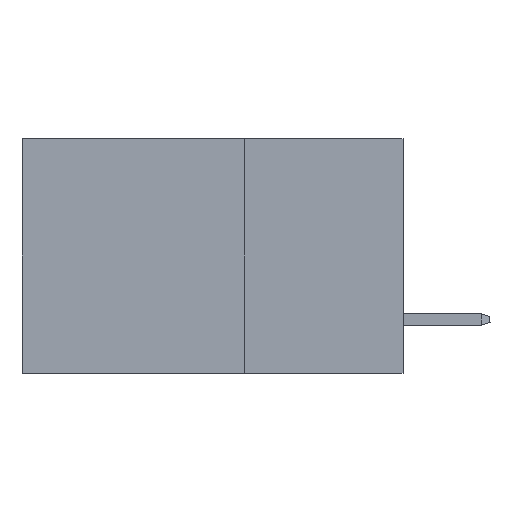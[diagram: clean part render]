
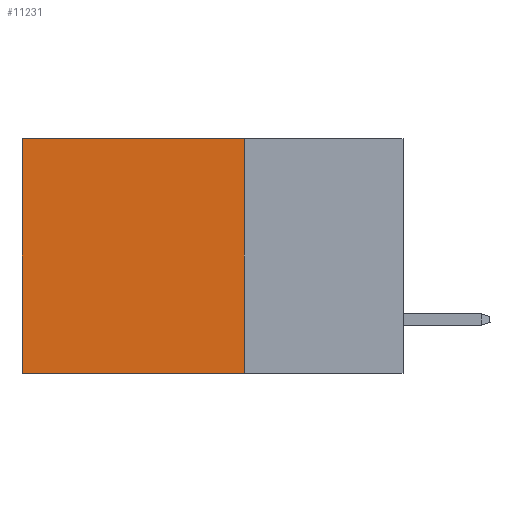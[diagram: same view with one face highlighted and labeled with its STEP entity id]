
A CAD part, left-side view. The second image highlights one B-rep face of the part: STEP entity #11231.
In plain terms, the highlighted planar face has unit normal (-1, 0, 0).
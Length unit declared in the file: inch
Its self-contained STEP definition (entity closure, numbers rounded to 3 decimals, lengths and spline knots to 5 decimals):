
#786 = DIRECTION ( 'NONE',  ( 0., 1., 0. ) ) ;
#881 = CARTESIAN_POINT ( 'NONE',  ( 0.2875, 0.25, 0. ) ) ;
#2865 = ORIENTED_EDGE ( 'NONE', *, *, #5326, .T. ) ;
#2967 = CARTESIAN_POINT ( 'NONE',  ( 0.2875, 0.25, 0. ) ) ;
#3061 = DIRECTION ( 'NONE',  ( 0., 0., -1. ) ) ;
#3342 = EDGE_CURVE ( 'NONE', #11267, #6676, #10036, .T. ) ;
#4133 = EDGE_CURVE ( 'NONE', #6849, #17588, #9976, .T. ) ;
#4524 = VECTOR ( 'NONE', #786, 39.37008 ) ;
#4807 = ORIENTED_EDGE ( 'NONE', *, *, #4133, .T. ) ;
#5004 = VECTOR ( 'NONE', #3061, 39.37008 ) ;
#5183 = LINE ( 'NONE', #5374, #15391 ) ;
#5257 = CARTESIAN_POINT ( 'NONE',  ( 0.2875, 0.25, 0. ) ) ;
#5326 = EDGE_CURVE ( 'NONE', #17588, #6676, #5183, .T. ) ;
#5374 = CARTESIAN_POINT ( 'NONE',  ( 0.2875, 0.6, 0. ) ) ;
#6676 = VERTEX_POINT ( 'NONE', #10835 ) ;
#6849 = VERTEX_POINT ( 'NONE', #5257 ) ;
#7529 = VECTOR ( 'NONE', #11526, 39.37008 ) ;
#7548 = AXIS2_PLACEMENT_3D ( 'NONE', #2967, #9135, #13284 ) ;
#9087 = ORIENTED_EDGE ( 'NONE', *, *, #12196, .F. ) ;
#9135 = DIRECTION ( 'NONE',  ( 1., 0., 0. ) ) ;
#9141 = ORIENTED_EDGE ( 'NONE', *, *, #3342, .F. ) ;
#9976 = LINE ( 'NONE', #881, #4524 ) ;
#10036 = LINE ( 'NONE', #16179, #7529 ) ;
#10648 = FACE_OUTER_BOUND ( 'NONE', #15523, .T. ) ;
#10835 = CARTESIAN_POINT ( 'NONE',  ( 0.2875, 0.6, -0.37 ) ) ;
#11231 = ADVANCED_FACE ( 'NONE', ( #10648 ), #16810, .F. ) ;
#11267 = VERTEX_POINT ( 'NONE', #18519 ) ;
#11526 = DIRECTION ( 'NONE',  ( 0., 1., 0. ) ) ;
#12092 = CARTESIAN_POINT ( 'NONE',  ( 0.2875, 0.6, 0. ) ) ;
#12196 = EDGE_CURVE ( 'NONE', #6849, #11267, #18310, .T. ) ;
#13284 = DIRECTION ( 'NONE',  ( 0., 0., -1. ) ) ;
#14673 = DIRECTION ( 'NONE',  ( 0., 0., -1. ) ) ;
#15391 = VECTOR ( 'NONE', #14673, 39.37008 ) ;
#15523 = EDGE_LOOP ( 'NONE', ( #2865, #9141, #9087, #4807 ) ) ;
#16179 = CARTESIAN_POINT ( 'NONE',  ( 0.2875, 0.25, -0.37 ) ) ;
#16601 = CARTESIAN_POINT ( 'NONE',  ( 0.2875, 0.25, 0. ) ) ;
#16810 = PLANE ( 'NONE',  #7548 ) ;
#17588 = VERTEX_POINT ( 'NONE', #12092 ) ;
#18310 = LINE ( 'NONE', #16601, #5004 ) ;
#18519 = CARTESIAN_POINT ( 'NONE',  ( 0.2875, 0.25, -0.37 ) ) ;
